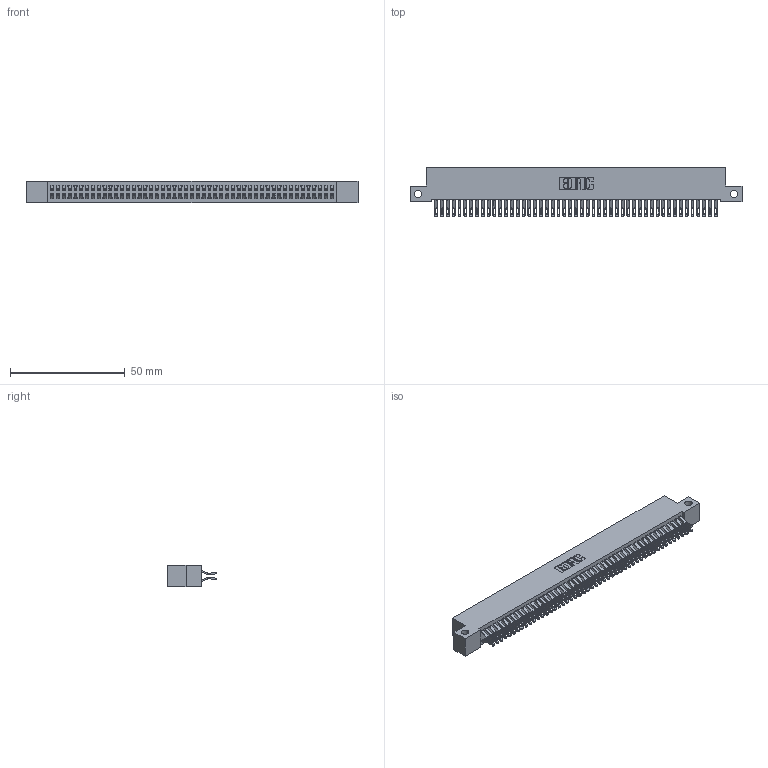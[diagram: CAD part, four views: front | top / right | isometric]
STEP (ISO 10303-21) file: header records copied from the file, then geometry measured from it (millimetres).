
FILE_DESCRIPTION (( 'STEP AP203' ), '1' );
FILE_NAME ('392-098-555-212.STEP', '2018-08-18T11:12:24', ( '' ), ( '' ), 'SwSTEP 2.0', 'SolidWorks 2016', '' );
FILE_SCHEMA (( 'CONFIG_CONTROL_DESIGN' ));
Length unit declared in the file: inch
Products named in the file (3): 342 Part_Side Mount; 345-292-001_555 Tail; 392-098-555-212
Assembly tree (99 placements, depth 2):
  392-098-555-212
    342 Part_Side Mount
    345-292-001_555 Tail  x98
Bounding box: 144.78 x 21.47 x 9.4 mm (x, y, z)
Volume: 13240 mm3; surface area: 22512.3 mm2
Topology: 99 solids, 99 shells, 5794 faces, 18233 edges, 12154 vertices
Faces by surface type: plane 3398, cylinder 2396
Entity records: 30815 total; most frequent: CARTESIAN_POINT 5132, ORIENTED_EDGE 5038, DIRECTION 4343, EDGE_CURVE 2519, LINE 2371, VECTOR 2371, VERTEX_POINT 1678, AXIS2_PLACEMENT_3D 986
